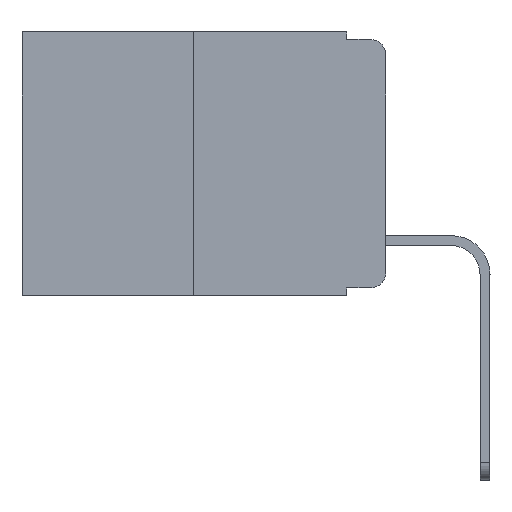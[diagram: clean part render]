
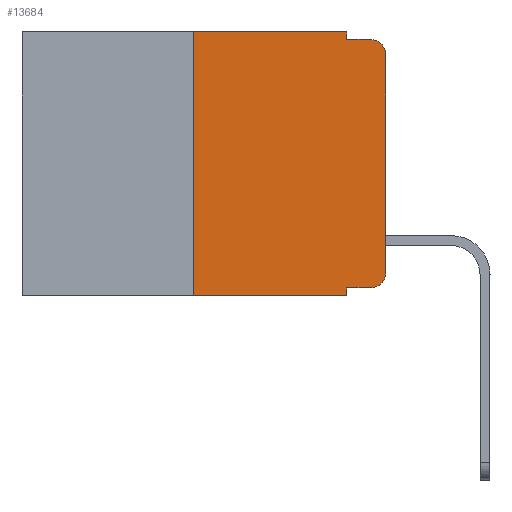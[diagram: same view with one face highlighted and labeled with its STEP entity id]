
A CAD part, left-side view. The second image highlights one B-rep face of the part: STEP entity #13684.
In plain terms, the highlighted planar face has unit normal (-1, 0, 0).
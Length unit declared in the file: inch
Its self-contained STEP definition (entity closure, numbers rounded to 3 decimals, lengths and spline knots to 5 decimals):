
#37 = ORIENTED_EDGE ( 'NONE', *, *, #15816, .T. ) ;
#795 = DIRECTION ( 'NONE',  ( 0., 0., -1. ) ) ;
#1305 = EDGE_CURVE ( 'NONE', #10277, #8021, #16575, .T. ) ;
#1584 = VECTOR ( 'NONE', #6506, 39.37008 ) ;
#1848 = LINE ( 'NONE', #7566, #12798 ) ;
#1940 = VERTEX_POINT ( 'NONE', #4948 ) ;
#2090 = ORIENTED_EDGE ( 'NONE', *, *, #11959, .F. ) ;
#2176 = EDGE_CURVE ( 'NONE', #15237, #11421, #2371, .T. ) ;
#2244 = LINE ( 'NONE', #14144, #5084 ) ;
#2365 = CARTESIAN_POINT ( 'NONE',  ( 0., 0., 0. ) ) ;
#2371 = CIRCLE ( 'NONE', #10262, 0.02 ) ;
#2806 = VECTOR ( 'NONE', #9741, 39.37008 ) ;
#3075 = EDGE_CURVE ( 'NONE', #11421, #1940, #13273, .T. ) ;
#3103 = CARTESIAN_POINT ( 'NONE',  ( 0., 0.25, -0.343 ) ) ;
#3382 = DIRECTION ( 'NONE',  ( -1., 0., 0. ) ) ;
#3501 = EDGE_CURVE ( 'NONE', #13412, #10277, #11667, .T. ) ;
#3821 = DIRECTION ( 'NONE',  ( -1., 0., 0. ) ) ;
#3941 = DIRECTION ( 'NONE',  ( 0., -1., 0. ) ) ;
#4134 = CARTESIAN_POINT ( 'NONE',  ( 0., 0.051, -0.01 ) ) ;
#4172 = FACE_OUTER_BOUND ( 'NONE', #15263, .T. ) ;
#4673 = CARTESIAN_POINT ( 'NONE',  ( 0., 0.473, 0. ) ) ;
#4948 = CARTESIAN_POINT ( 'NONE',  ( 0., 0., -0.03 ) ) ;
#4990 = VECTOR ( 'NONE', #15878, 39.37008 ) ;
#5022 = CARTESIAN_POINT ( 'NONE',  ( 0., 0.051, -0.343 ) ) ;
#5084 = VECTOR ( 'NONE', #3941, 39.37008 ) ;
#5218 = CARTESIAN_POINT ( 'NONE',  ( 0., 0.051, -0.01 ) ) ;
#5515 = DIRECTION ( 'NONE',  ( 0., -1., 0. ) ) ;
#5942 = AXIS2_PLACEMENT_3D ( 'NONE', #4673, #14991, #7287 ) ;
#6056 = CARTESIAN_POINT ( 'NONE',  ( 0., 0.051, 0. ) ) ;
#6168 = ORIENTED_EDGE ( 'NONE', *, *, #3075, .T. ) ;
#6243 = LINE ( 'NONE', #14735, #2806 ) ;
#6337 = CARTESIAN_POINT ( 'NONE',  ( 0., 0.02, -0.01 ) ) ;
#6506 = DIRECTION ( 'NONE',  ( 0., -1., 0. ) ) ;
#6901 = VERTEX_POINT ( 'NONE', #5022 ) ;
#6910 = CARTESIAN_POINT ( 'NONE',  ( 0., 0.25, 0. ) ) ;
#7287 = DIRECTION ( 'NONE',  ( 0., 0., -1. ) ) ;
#7554 = VERTEX_POINT ( 'NONE', #5218 ) ;
#7566 = CARTESIAN_POINT ( 'NONE',  ( 0., 0.051, 0. ) ) ;
#7763 = CARTESIAN_POINT ( 'NONE',  ( 0., 0.051, -0.333 ) ) ;
#7803 = DIRECTION ( 'NONE',  ( 0., 0., -1. ) ) ;
#7876 = ORIENTED_EDGE ( 'NONE', *, *, #2176, .T. ) ;
#8021 = VERTEX_POINT ( 'NONE', #6056 ) ;
#8612 = CARTESIAN_POINT ( 'NONE',  ( 0., 0.25, 0. ) ) ;
#8835 = VERTEX_POINT ( 'NONE', #7763 ) ;
#9163 = ORIENTED_EDGE ( 'NONE', *, *, #1305, .F. ) ;
#9304 = DIRECTION ( 'NONE',  ( 0., -1., 0. ) ) ;
#9375 = EDGE_CURVE ( 'NONE', #13412, #6901, #2244, .T. ) ;
#9741 = DIRECTION ( 'NONE',  ( 0., 0., -1. ) ) ;
#9827 = AXIS2_PLACEMENT_3D ( 'NONE', #11121, #3382, #12423 ) ;
#9872 = VECTOR ( 'NONE', #10199, 39.37008 ) ;
#10199 = DIRECTION ( 'NONE',  ( 0., 0., 1. ) ) ;
#10255 = CARTESIAN_POINT ( 'NONE',  ( 0., 0., -0.313 ) ) ;
#10262 = AXIS2_PLACEMENT_3D ( 'NONE', #11224, #3821, #7803 ) ;
#10277 = VERTEX_POINT ( 'NONE', #8612 ) ;
#10356 = LINE ( 'NONE', #15833, #13362 ) ;
#11121 = CARTESIAN_POINT ( 'NONE',  ( 0., 0.02, -0.03 ) ) ;
#11224 = CARTESIAN_POINT ( 'NONE',  ( 0., 0.02, -0.313 ) ) ;
#11234 = LINE ( 'NONE', #4134, #15893 ) ;
#11421 = VERTEX_POINT ( 'NONE', #10255 ) ;
#11667 = LINE ( 'NONE', #6910, #4990 ) ;
#11959 = EDGE_CURVE ( 'NONE', #8835, #6901, #6243, .T. ) ;
#12166 = VERTEX_POINT ( 'NONE', #6337 ) ;
#12423 = DIRECTION ( 'NONE',  ( 0., 0., -1. ) ) ;
#12728 = ORIENTED_EDGE ( 'NONE', *, *, #16417, .F. ) ;
#12798 = VECTOR ( 'NONE', #795, 39.37008 ) ;
#13273 = LINE ( 'NONE', #2365, #9872 ) ;
#13354 = ORIENTED_EDGE ( 'NONE', *, *, #9375, .T. ) ;
#13362 = VECTOR ( 'NONE', #9304, 39.37008 ) ;
#13412 = VERTEX_POINT ( 'NONE', #3103 ) ;
#13422 = EDGE_CURVE ( 'NONE', #7554, #12166, #11234, .T. ) ;
#13684 = ADVANCED_FACE ( 'NONE', ( #4172 ), #13849, .F. ) ;
#13849 = PLANE ( 'NONE',  #5942 ) ;
#14024 = CIRCLE ( 'NONE', #9827, 0.02 ) ;
#14055 = CARTESIAN_POINT ( 'NONE',  ( 0., 0.473, 0. ) ) ;
#14144 = CARTESIAN_POINT ( 'NONE',  ( 0., 0.473, -0.343 ) ) ;
#14593 = ORIENTED_EDGE ( 'NONE', *, *, #3501, .F. ) ;
#14735 = CARTESIAN_POINT ( 'NONE',  ( 0., 0.051, 0. ) ) ;
#14991 = DIRECTION ( 'NONE',  ( 1., 0., 0. ) ) ;
#15237 = VERTEX_POINT ( 'NONE', #16250 ) ;
#15263 = EDGE_LOOP ( 'NONE', ( #6168, #37, #15394, #12728, #9163, #14593, #13354, #2090, #15514, #7876 ) ) ;
#15394 = ORIENTED_EDGE ( 'NONE', *, *, #13422, .F. ) ;
#15514 = ORIENTED_EDGE ( 'NONE', *, *, #15534, .T. ) ;
#15534 = EDGE_CURVE ( 'NONE', #8835, #15237, #10356, .T. ) ;
#15816 = EDGE_CURVE ( 'NONE', #1940, #12166, #14024, .T. ) ;
#15833 = CARTESIAN_POINT ( 'NONE',  ( 0., 0.051, -0.333 ) ) ;
#15878 = DIRECTION ( 'NONE',  ( 0., 0., 1. ) ) ;
#15893 = VECTOR ( 'NONE', #5515, 39.37008 ) ;
#16250 = CARTESIAN_POINT ( 'NONE',  ( 0., 0.02, -0.333 ) ) ;
#16417 = EDGE_CURVE ( 'NONE', #8021, #7554, #1848, .T. ) ;
#16575 = LINE ( 'NONE', #14055, #1584 ) ;
